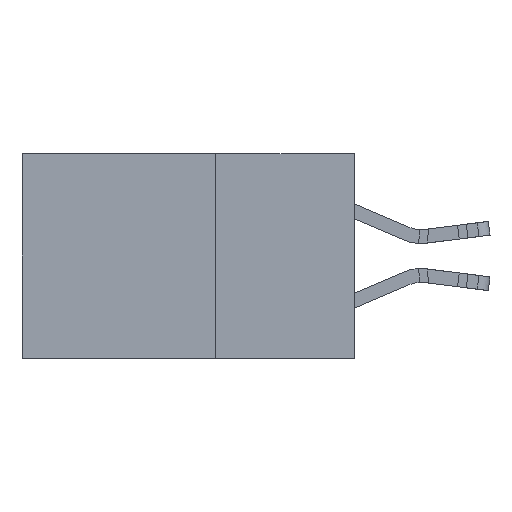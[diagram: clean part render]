
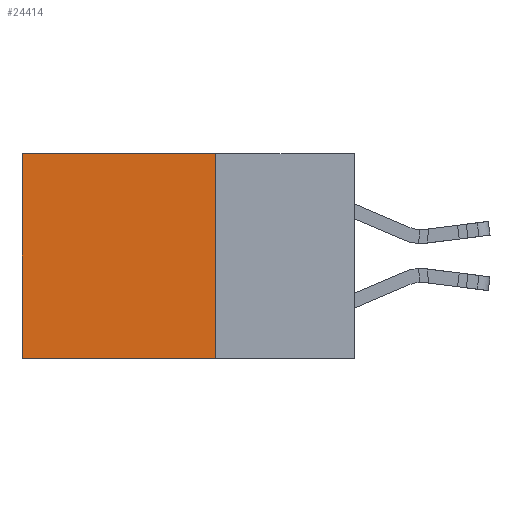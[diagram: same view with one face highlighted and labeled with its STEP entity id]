
A CAD part, left-side view. The second image highlights one B-rep face of the part: STEP entity #24414.
In plain terms, the highlighted planar face has unit normal (-1, 0, 0).
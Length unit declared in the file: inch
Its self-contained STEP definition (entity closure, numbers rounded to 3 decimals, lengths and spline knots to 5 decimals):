
#407 = VECTOR ( 'NONE', #28788, 39.37008 ) ;
#2617 = EDGE_CURVE ( 'NONE', #21806, #19801, #19670, .T. ) ;
#4304 = AXIS2_PLACEMENT_3D ( 'NONE', #30456, #5702, #23175 ) ;
#5702 = DIRECTION ( 'NONE',  ( 1., 0., 0. ) ) ;
#8172 = CARTESIAN_POINT ( 'NONE',  ( 0.298, 0.25, -0.37 ) ) ;
#8245 = FACE_OUTER_BOUND ( 'NONE', #21589, .T. ) ;
#8513 = VECTOR ( 'NONE', #31001, 39.37008 ) ;
#9976 = ORIENTED_EDGE ( 'NONE', *, *, #24606, .T. ) ;
#10338 = DIRECTION ( 'NONE',  ( 0., 1., 0. ) ) ;
#11340 = CARTESIAN_POINT ( 'NONE',  ( 0.298, 0.25, 0. ) ) ;
#13433 = VERTEX_POINT ( 'NONE', #30901 ) ;
#13704 = LINE ( 'NONE', #16342, #407 ) ;
#14478 = VECTOR ( 'NONE', #16302, 39.37008 ) ;
#15027 = ORIENTED_EDGE ( 'NONE', *, *, #31892, .T. ) ;
#15983 = ORIENTED_EDGE ( 'NONE', *, *, #17289, .F. ) ;
#16302 = DIRECTION ( 'NONE',  ( 0., 1., 0. ) ) ;
#16342 = CARTESIAN_POINT ( 'NONE',  ( 0.298, 0.6, 0. ) ) ;
#17289 = EDGE_CURVE ( 'NONE', #29154, #21806, #21773, .T. ) ;
#18285 = CARTESIAN_POINT ( 'NONE',  ( 0.298, 0.25, -0.37 ) ) ;
#19493 = CARTESIAN_POINT ( 'NONE',  ( 0.298, 0.25, 0. ) ) ;
#19670 = LINE ( 'NONE', #18285, #31966 ) ;
#19801 = VERTEX_POINT ( 'NONE', #24232 ) ;
#20667 = PLANE ( 'NONE',  #4304 ) ;
#21589 = EDGE_LOOP ( 'NONE', ( #15027, #30076, #15983, #9976 ) ) ;
#21773 = LINE ( 'NONE', #26100, #8513 ) ;
#21806 = VERTEX_POINT ( 'NONE', #8172 ) ;
#23175 = DIRECTION ( 'NONE',  ( 0., 0., -1. ) ) ;
#24232 = CARTESIAN_POINT ( 'NONE',  ( 0.298, 0.6, -0.37 ) ) ;
#24414 = ADVANCED_FACE ( 'NONE', ( #8245 ), #20667, .F. ) ;
#24606 = EDGE_CURVE ( 'NONE', #29154, #13433, #27667, .T. ) ;
#26100 = CARTESIAN_POINT ( 'NONE',  ( 0.298, 0.25, 0. ) ) ;
#27667 = LINE ( 'NONE', #11340, #14478 ) ;
#28788 = DIRECTION ( 'NONE',  ( 0., 0., -1. ) ) ;
#29154 = VERTEX_POINT ( 'NONE', #19493 ) ;
#30076 = ORIENTED_EDGE ( 'NONE', *, *, #2617, .F. ) ;
#30456 = CARTESIAN_POINT ( 'NONE',  ( 0.298, 0.25, 0. ) ) ;
#30901 = CARTESIAN_POINT ( 'NONE',  ( 0.298, 0.6, 0. ) ) ;
#31001 = DIRECTION ( 'NONE',  ( 0., 0., -1. ) ) ;
#31892 = EDGE_CURVE ( 'NONE', #13433, #19801, #13704, .T. ) ;
#31966 = VECTOR ( 'NONE', #10338, 39.37008 ) ;
